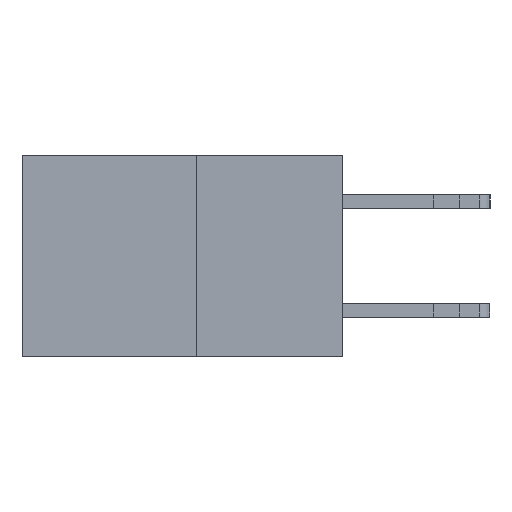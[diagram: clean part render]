
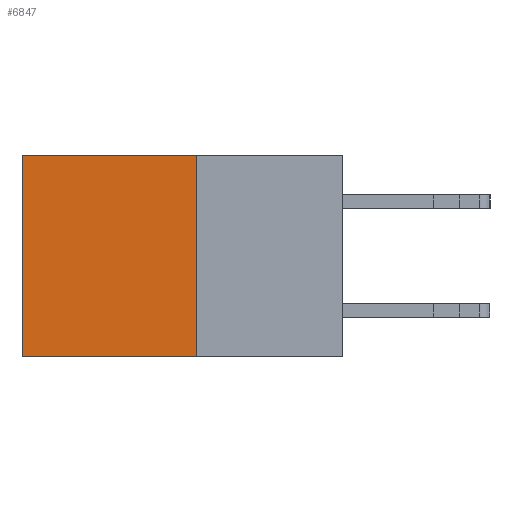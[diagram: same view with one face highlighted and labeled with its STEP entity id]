
A CAD part, left-side view. The second image highlights one B-rep face of the part: STEP entity #6847.
In plain terms, the highlighted planar face has unit normal (-1, 0, 0).
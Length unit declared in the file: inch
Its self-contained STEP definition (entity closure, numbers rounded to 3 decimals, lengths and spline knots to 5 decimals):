
#59 = LINE ( 'NONE', #5876, #5590 ) ;
#740 = EDGE_CURVE ( 'NONE', #1858, #12866, #2218, .T. ) ;
#1824 = CARTESIAN_POINT ( 'NONE',  ( 0.277, 0.27, 0. ) ) ;
#1858 = VERTEX_POINT ( 'NONE', #12506 ) ;
#2218 = LINE ( 'NONE', #3820, #13678 ) ;
#2440 = FACE_OUTER_BOUND ( 'NONE', #12411, .T. ) ;
#3294 = CARTESIAN_POINT ( 'NONE',  ( 0.277, 0.59, 0. ) ) ;
#3326 = VECTOR ( 'NONE', #13472, 39.37008 ) ;
#3656 = DIRECTION ( 'NONE',  ( 0., 1., 0. ) ) ;
#3820 = CARTESIAN_POINT ( 'NONE',  ( 0.277, 0.27, -0.37 ) ) ;
#4719 = CARTESIAN_POINT ( 'NONE',  ( 0.277, 0.59, -0.37 ) ) ;
#5013 = CARTESIAN_POINT ( 'NONE',  ( 0.277, 0.59, -0.37 ) ) ;
#5263 = LINE ( 'NONE', #1824, #11139 ) ;
#5413 = CARTESIAN_POINT ( 'NONE',  ( 0.277, 0.27, -0.37 ) ) ;
#5590 = VECTOR ( 'NONE', #3656, 39.37008 ) ;
#5876 = CARTESIAN_POINT ( 'NONE',  ( 0.277, 0.27, -0.37 ) ) ;
#6313 = CARTESIAN_POINT ( 'NONE',  ( 0.277, 0.27, -0.37 ) ) ;
#6458 = PLANE ( 'NONE',  #11809 ) ;
#6847 = ADVANCED_FACE ( 'NONE', ( #2440 ), #6458, .F. ) ;
#7498 = ORIENTED_EDGE ( 'NONE', *, *, #12779, .T. ) ;
#8608 = DIRECTION ( 'NONE',  ( 0., 1., 0. ) ) ;
#9033 = VERTEX_POINT ( 'NONE', #5013 ) ;
#9381 = DIRECTION ( 'NONE',  ( 1., 0., 0. ) ) ;
#9642 = LINE ( 'NONE', #4719, #3326 ) ;
#10573 = ORIENTED_EDGE ( 'NONE', *, *, #13155, .F. ) ;
#10773 = VERTEX_POINT ( 'NONE', #3294 ) ;
#11135 = DIRECTION ( 'NONE',  ( 0., 0., -1. ) ) ;
#11139 = VECTOR ( 'NONE', #8608, 39.37008 ) ;
#11427 = EDGE_CURVE ( 'NONE', #10773, #9033, #9642, .T. ) ;
#11809 = AXIS2_PLACEMENT_3D ( 'NONE', #6313, #9381, #14139 ) ;
#12411 = EDGE_LOOP ( 'NONE', ( #13223, #10573, #13603, #7498 ) ) ;
#12506 = CARTESIAN_POINT ( 'NONE',  ( 0.277, 0.27, 0. ) ) ;
#12779 = EDGE_CURVE ( 'NONE', #1858, #10773, #5263, .T. ) ;
#12866 = VERTEX_POINT ( 'NONE', #5413 ) ;
#13155 = EDGE_CURVE ( 'NONE', #12866, #9033, #59, .T. ) ;
#13223 = ORIENTED_EDGE ( 'NONE', *, *, #11427, .T. ) ;
#13472 = DIRECTION ( 'NONE',  ( 0., 0., -1. ) ) ;
#13603 = ORIENTED_EDGE ( 'NONE', *, *, #740, .F. ) ;
#13678 = VECTOR ( 'NONE', #11135, 39.37008 ) ;
#14139 = DIRECTION ( 'NONE',  ( 0., 0., -1. ) ) ;
